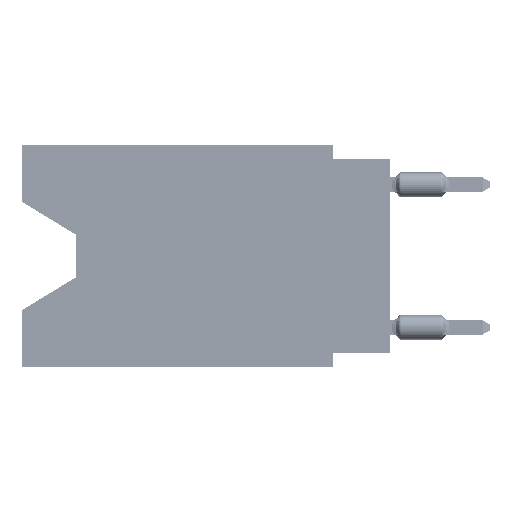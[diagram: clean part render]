
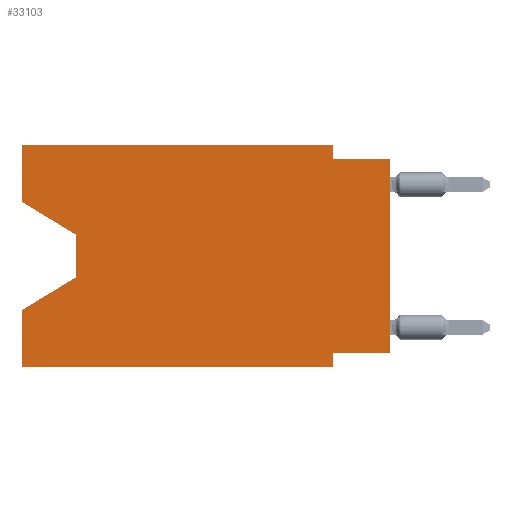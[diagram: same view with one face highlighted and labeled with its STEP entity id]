
A CAD part, left-side view. The second image highlights one B-rep face of the part: STEP entity #33103.
In plain terms, the highlighted planar face has unit normal (-1, 0, 0).
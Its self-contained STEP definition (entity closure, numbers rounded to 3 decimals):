
#179 = VECTOR ( 'NONE', #33216, 1000. ) ;
#609 = VERTEX_POINT ( 'NONE', #36622 ) ;
#831 = EDGE_LOOP ( 'NONE', ( #15855, #44828, #37198, #37315, #39976, #5140, #55069, #12843, #20779, #53803, #14809, #16921 ) ) ;
#1554 = VERTEX_POINT ( 'NONE', #8510 ) ;
#1912 = CARTESIAN_POINT ( 'NONE',  ( 0., 13.97, -5.893 ) ) ;
#2064 = CARTESIAN_POINT ( 'NONE',  ( 0., 2.54, -0.635 ) ) ;
#2210 = EDGE_CURVE ( 'NONE', #58439, #17440, #22114, .T. ) ;
#3248 = LINE ( 'NONE', #1912, #12471 ) ;
#3290 = VERTEX_POINT ( 'NONE', #56413 ) ;
#4068 = CARTESIAN_POINT ( 'NONE',  ( 0., 2.54, -9.906 ) ) ;
#4959 = VECTOR ( 'NONE', #27031, 1000. ) ;
#5140 = ORIENTED_EDGE ( 'NONE', *, *, #62933, .F. ) ;
#5291 = DIRECTION ( 'NONE',  ( 0., 0., -1. ) ) ;
#6006 = CARTESIAN_POINT ( 'NONE',  ( 0., 16.383, 0. ) ) ;
#6059 = VERTEX_POINT ( 'NONE', #27995 ) ;
#8129 = LINE ( 'NONE', #12279, #179 ) ;
#8274 = DIRECTION ( 'NONE',  ( 0., 0., 1. ) ) ;
#8510 = CARTESIAN_POINT ( 'NONE',  ( 0., 13.97, -5.893 ) ) ;
#8717 = EDGE_CURVE ( 'NONE', #609, #31335, #8129, .T. ) ;
#9066 = VECTOR ( 'NONE', #8274, 1000. ) ;
#9371 = DIRECTION ( 'NONE',  ( 0., -1., 0. ) ) ;
#10314 = VERTEX_POINT ( 'NONE', #32229 ) ;
#11345 = CARTESIAN_POINT ( 'NONE',  ( 0., 16.383, 0. ) ) ;
#11910 = LINE ( 'NONE', #27690, #4959 ) ;
#12279 = CARTESIAN_POINT ( 'NONE',  ( 0., 0., -9.271 ) ) ;
#12471 = VECTOR ( 'NONE', #44111, 1000. ) ;
#12774 = VECTOR ( 'NONE', #16644, 1000. ) ;
#12843 = ORIENTED_EDGE ( 'NONE', *, *, #24206, .T. ) ;
#13030 = LINE ( 'NONE', #54904, #54809 ) ;
#13363 = EDGE_CURVE ( 'NONE', #3290, #1554, #13030, .T. ) ;
#14104 = EDGE_CURVE ( 'NONE', #1554, #10314, #3248, .T. ) ;
#14809 = ORIENTED_EDGE ( 'NONE', *, *, #2210, .F. ) ;
#15855 = ORIENTED_EDGE ( 'NONE', *, *, #45674, .T. ) ;
#16644 = DIRECTION ( 'NONE',  ( 0., 0., 1. ) ) ;
#16921 = ORIENTED_EDGE ( 'NONE', *, *, #64825, .F. ) ;
#17394 = VECTOR ( 'NONE', #9371, 1000. ) ;
#17440 = VERTEX_POINT ( 'NONE', #52902 ) ;
#19144 = EDGE_CURVE ( 'NONE', #41782, #10314, #27146, .T. ) ;
#19674 = CARTESIAN_POINT ( 'NONE',  ( 0., 0., -0.635 ) ) ;
#20522 = DIRECTION ( 'NONE',  ( 0., 0., -1. ) ) ;
#20779 = ORIENTED_EDGE ( 'NONE', *, *, #51457, .F. ) ;
#21122 = CARTESIAN_POINT ( 'NONE',  ( 0., 16.383, 0. ) ) ;
#22114 = LINE ( 'NONE', #63995, #51708 ) ;
#23417 = PLANE ( 'NONE',  #34534 ) ;
#23729 = CARTESIAN_POINT ( 'NONE',  ( 0., 0., 0. ) ) ;
#24206 = EDGE_CURVE ( 'NONE', #609, #39372, #55647, .T. ) ;
#24426 = FACE_OUTER_BOUND ( 'NONE', #831, .T. ) ;
#27031 = DIRECTION ( 'NONE',  ( 0., -0.855, -0.519 ) ) ;
#27146 = LINE ( 'NONE', #11345, #57272 ) ;
#27281 = DIRECTION ( 'NONE',  ( 0., -1., 0. ) ) ;
#27690 = CARTESIAN_POINT ( 'NONE',  ( 0., 16.383, -2.546 ) ) ;
#27995 = CARTESIAN_POINT ( 'NONE',  ( 0., 2.54, -9.906 ) ) ;
#30479 = VERTEX_POINT ( 'NONE', #2064 ) ;
#31335 = VERTEX_POINT ( 'NONE', #59209 ) ;
#31505 = EDGE_CURVE ( 'NONE', #17440, #30479, #56420, .T. ) ;
#32229 = CARTESIAN_POINT ( 'NONE',  ( 0., 16.383, -7.36 ) ) ;
#33103 = ADVANCED_FACE ( 'NONE', ( #24426 ), #23417, .F. ) ;
#33216 = DIRECTION ( 'NONE',  ( 0., 1., 0. ) ) ;
#33640 = VERTEX_POINT ( 'NONE', #47609 ) ;
#34534 = AXIS2_PLACEMENT_3D ( 'NONE', #44375, #65311, #47100 ) ;
#35477 = VECTOR ( 'NONE', #5291, 1000. ) ;
#35663 = VECTOR ( 'NONE', #20522, 1000. ) ;
#36622 = CARTESIAN_POINT ( 'NONE',  ( 0., 0., -9.271 ) ) ;
#37116 = DIRECTION ( 'NONE',  ( 0., 0., 1. ) ) ;
#37198 = ORIENTED_EDGE ( 'NONE', *, *, #14104, .T. ) ;
#37315 = ORIENTED_EDGE ( 'NONE', *, *, #19144, .F. ) ;
#39346 = CARTESIAN_POINT ( 'NONE',  ( 0., 0., -0.635 ) ) ;
#39372 = VERTEX_POINT ( 'NONE', #39346 ) ;
#39976 = ORIENTED_EDGE ( 'NONE', *, *, #63593, .T. ) ;
#40287 = LINE ( 'NONE', #19674, #17394 ) ;
#41782 = VERTEX_POINT ( 'NONE', #45877 ) ;
#44111 = DIRECTION ( 'NONE',  ( 0., 0.855, -0.519 ) ) ;
#44375 = CARTESIAN_POINT ( 'NONE',  ( 0., 16.383, 0. ) ) ;
#44828 = ORIENTED_EDGE ( 'NONE', *, *, #13363, .T. ) ;
#45674 = EDGE_CURVE ( 'NONE', #33640, #3290, #11910, .T. ) ;
#45877 = CARTESIAN_POINT ( 'NONE',  ( 0., 16.383, -9.906 ) ) ;
#46889 = LINE ( 'NONE', #63338, #52188 ) ;
#47100 = DIRECTION ( 'NONE',  ( 0., 0., -1. ) ) ;
#47609 = CARTESIAN_POINT ( 'NONE',  ( 0., 16.383, -2.546 ) ) ;
#50773 = DIRECTION ( 'NONE',  ( 0., 0., -1. ) ) ;
#51457 = EDGE_CURVE ( 'NONE', #30479, #39372, #40287, .T. ) ;
#51621 = CARTESIAN_POINT ( 'NONE',  ( 0., 2.54, 0. ) ) ;
#51708 = VECTOR ( 'NONE', #27281, 1000. ) ;
#52188 = VECTOR ( 'NONE', #53020, 1000. ) ;
#52902 = CARTESIAN_POINT ( 'NONE',  ( 0., 2.54, 0. ) ) ;
#53020 = DIRECTION ( 'NONE',  ( 0., -1., 0. ) ) ;
#53803 = ORIENTED_EDGE ( 'NONE', *, *, #31505, .F. ) ;
#54809 = VECTOR ( 'NONE', #50773, 1000. ) ;
#54904 = CARTESIAN_POINT ( 'NONE',  ( 0., 13.97, -4.013 ) ) ;
#55069 = ORIENTED_EDGE ( 'NONE', *, *, #8717, .F. ) ;
#55647 = LINE ( 'NONE', #23729, #9066 ) ;
#56413 = CARTESIAN_POINT ( 'NONE',  ( 0., 13.97, -4.013 ) ) ;
#56420 = LINE ( 'NONE', #51621, #35477 ) ;
#56901 = LINE ( 'NONE', #4068, #35663 ) ;
#57272 = VECTOR ( 'NONE', #37116, 1000. ) ;
#58439 = VERTEX_POINT ( 'NONE', #6006 ) ;
#59209 = CARTESIAN_POINT ( 'NONE',  ( 0., 2.54, -9.271 ) ) ;
#62933 = EDGE_CURVE ( 'NONE', #31335, #6059, #56901, .T. ) ;
#63338 = CARTESIAN_POINT ( 'NONE',  ( 0., 16.383, -9.906 ) ) ;
#63593 = EDGE_CURVE ( 'NONE', #41782, #6059, #46889, .T. ) ;
#63676 = LINE ( 'NONE', #21122, #12774 ) ;
#63995 = CARTESIAN_POINT ( 'NONE',  ( 0., 16.383, 0. ) ) ;
#64825 = EDGE_CURVE ( 'NONE', #33640, #58439, #63676, .T. ) ;
#65311 = DIRECTION ( 'NONE',  ( 1., 0., 0. ) ) ;
